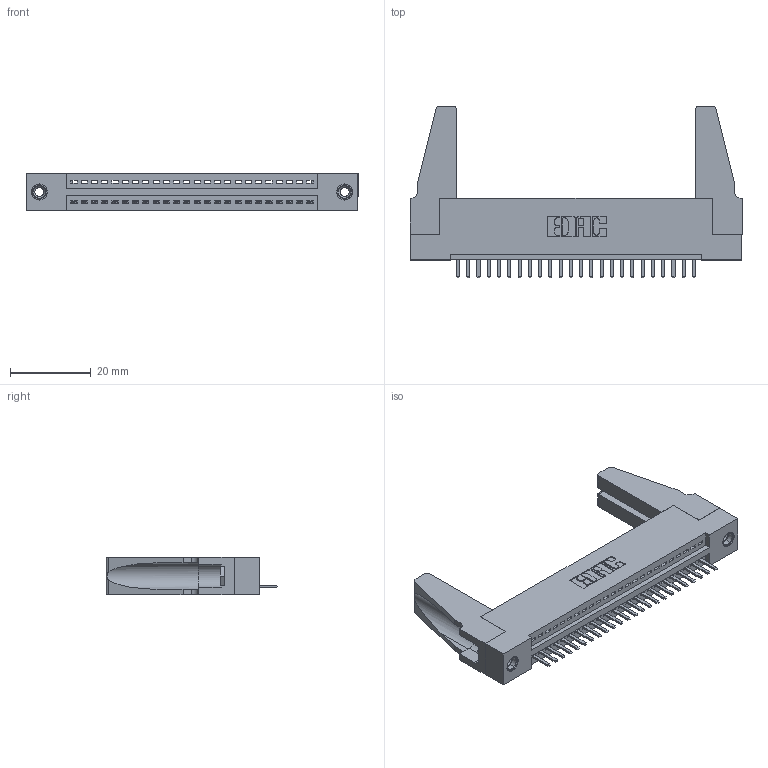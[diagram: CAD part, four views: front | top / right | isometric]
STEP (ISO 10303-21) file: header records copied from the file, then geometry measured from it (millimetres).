
FILE_DESCRIPTION (( 'STEP AP203' ), '1' );
FILE_NAME ('345-024-520-188.STEP', '2019-10-05T03:41:36', ( '' ), ( '' ), 'SwSTEP 2.0', 'SolidWorks 2016', '' );
FILE_SCHEMA (( 'CONFIG_CONTROL_DESIGN' ));
Length unit declared in the file: inch
Products named in the file (5): 345-250-001_345-250-001-102; 345 Part_Flush Mounting Lugs - 0.156 Dia-TH; 345-024-520-188; 345-292-001_345-293-120; 345-220-078_345-220-088
Assembly tree (29 placements, depth 2):
  345-024-520-188
    345 Part_Flush Mounting Lugs - 0.156 Dia-TH
    345-292-001_345-293-120  x24
    345-250-001_345-250-001-102  x2
    345-220-078_345-220-088  x2
Bounding box: 82.19 x 42.55 x 9.4 mm (x, y, z)
Volume: 10842.9 mm3; surface area: 12745.8 mm2
Topology: 29 solids, 29 shells, 1738 faces, 5071 edges, 3306 vertices
Faces by surface type: plane 1160, cylinder 562, cone 12, torus 4
Entity records: 22748 total; most frequent: CARTESIAN_POINT 3942, ORIENTED_EDGE 3848, DIRECTION 3464, EDGE_CURVE 1924, VECTOR 1650, LINE 1650, VERTEX_POINT 1274, AXIS2_PLACEMENT_3D 907
